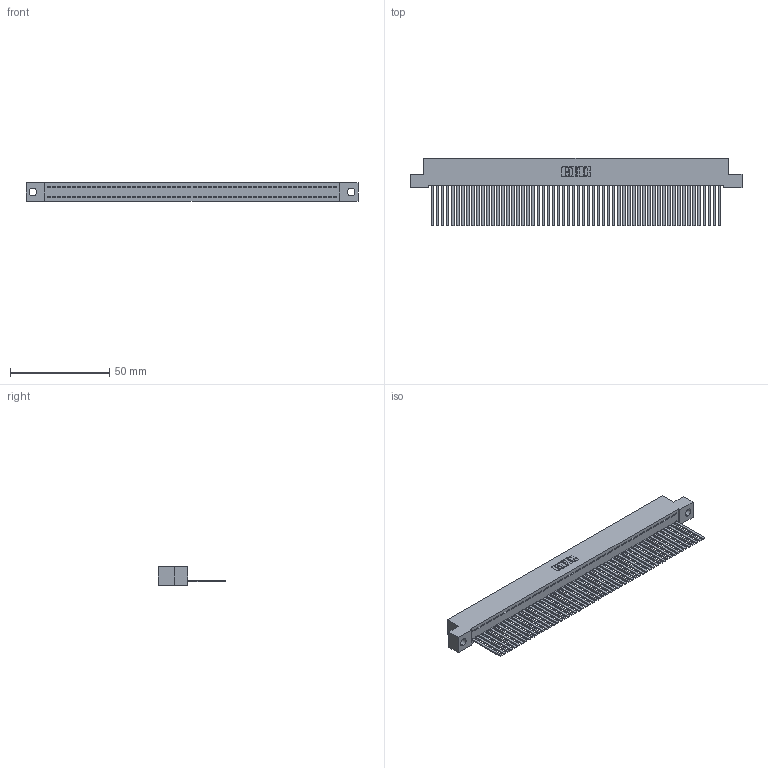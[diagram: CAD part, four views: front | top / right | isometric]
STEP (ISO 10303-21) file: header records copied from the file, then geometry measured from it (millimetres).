
FILE_DESCRIPTION (( 'STEP AP203' ), '1' );
FILE_NAME ('342-058-544-104.STEP', '2018-08-13T05:30:45', ( '' ), ( '' ), 'SwSTEP 2.0', 'SolidWorks 2016', '' );
FILE_SCHEMA (( 'CONFIG_CONTROL_DESIGN' ));
Length unit declared in the file: inch
Products named in the file (3): 342 Part_.156 TH; 345-292-001_345-293-144; 342-058-544-104
Assembly tree (59 placements, depth 2):
  342-058-544-104
    342 Part_.156 TH
    345-292-001_345-293-144  x58
Bounding box: 167.64 x 34.3 x 9.4 mm (x, y, z)
Volume: 15342.3 mm3; surface area: 24558.8 mm2
Topology: 59 solids, 59 shells, 3126 faces, 9463 edges, 6230 vertices
Faces by surface type: plane 2270, cylinder 856
Entity records: 33075 total; most frequent: CARTESIAN_POINT 5708, ORIENTED_EDGE 5702, DIRECTION 4779, EDGE_CURVE 2851, LINE 2727, VECTOR 2727, VERTEX_POINT 1898, AXIS2_PLACEMENT_3D 1026
